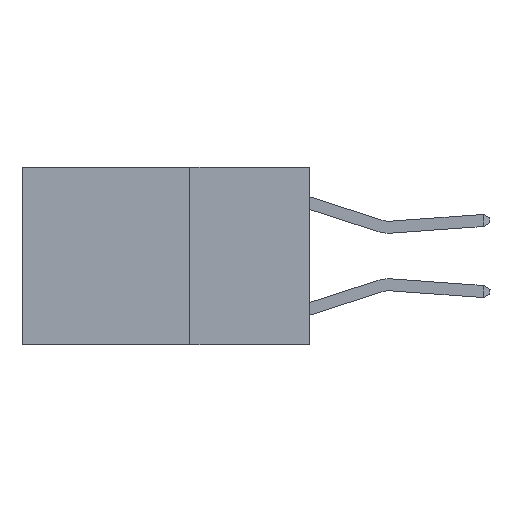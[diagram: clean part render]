
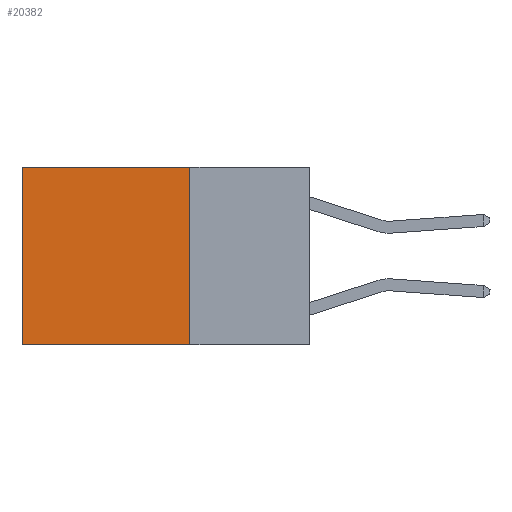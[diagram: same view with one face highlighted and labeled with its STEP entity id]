
A CAD part, left-side view. The second image highlights one B-rep face of the part: STEP entity #20382.
In plain terms, the highlighted planar face has unit normal (-1, 0, 0).
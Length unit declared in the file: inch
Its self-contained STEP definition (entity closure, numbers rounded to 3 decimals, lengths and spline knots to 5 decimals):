
#533 = VERTEX_POINT ( 'NONE', #4999 ) ;
#788 = PLANE ( 'NONE',  #25229 ) ;
#1667 = LINE ( 'NONE', #12451, #21336 ) ;
#1878 = LINE ( 'NONE', #17025, #21306 ) ;
#2861 = LINE ( 'NONE', #4998, #4968 ) ;
#3284 = EDGE_LOOP ( 'NONE', ( #20210, #12112, #8205, #14274 ) ) ;
#3527 = LINE ( 'NONE', #20794, #27763 ) ;
#4647 = EDGE_CURVE ( 'NONE', #10671, #533, #1667, .T. ) ;
#4968 = VECTOR ( 'NONE', #11514, 39.37008 ) ;
#4998 = CARTESIAN_POINT ( 'NONE',  ( 0.2625, 0.6, 0. ) ) ;
#4999 = CARTESIAN_POINT ( 'NONE',  ( 0.2625, 0.25, -0.37 ) ) ;
#8091 = EDGE_CURVE ( 'NONE', #10671, #26003, #1878, .T. ) ;
#8205 = ORIENTED_EDGE ( 'NONE', *, *, #4647, .F. ) ;
#10469 = DIRECTION ( 'NONE',  ( 0., 1., 0. ) ) ;
#10671 = VERTEX_POINT ( 'NONE', #18502 ) ;
#10900 = CARTESIAN_POINT ( 'NONE',  ( 0.2625, 0.6, 0. ) ) ;
#11514 = DIRECTION ( 'NONE',  ( 0., 0., -1. ) ) ;
#12112 = ORIENTED_EDGE ( 'NONE', *, *, #27136, .F. ) ;
#12451 = CARTESIAN_POINT ( 'NONE',  ( 0.2625, 0.25, 0. ) ) ;
#13830 = CARTESIAN_POINT ( 'NONE',  ( 0.2625, 0.25, 0. ) ) ;
#14274 = ORIENTED_EDGE ( 'NONE', *, *, #8091, .T. ) ;
#15683 = FACE_OUTER_BOUND ( 'NONE', #3284, .T. ) ;
#17025 = CARTESIAN_POINT ( 'NONE',  ( 0.2625, 0.25, 0. ) ) ;
#17937 = DIRECTION ( 'NONE',  ( 0., 0., -1. ) ) ;
#18502 = CARTESIAN_POINT ( 'NONE',  ( 0.2625, 0.25, 0. ) ) ;
#20210 = ORIENTED_EDGE ( 'NONE', *, *, #22413, .T. ) ;
#20382 = ADVANCED_FACE ( 'NONE', ( #15683 ), #788, .F. ) ;
#20794 = CARTESIAN_POINT ( 'NONE',  ( 0.2625, 0.25, -0.37 ) ) ;
#21072 = DIRECTION ( 'NONE',  ( 0., 0., -1. ) ) ;
#21224 = CARTESIAN_POINT ( 'NONE',  ( 0.2625, 0.6, -0.37 ) ) ;
#21306 = VECTOR ( 'NONE', #25677, 39.37008 ) ;
#21336 = VECTOR ( 'NONE', #21072, 39.37008 ) ;
#21761 = VERTEX_POINT ( 'NONE', #21224 ) ;
#22413 = EDGE_CURVE ( 'NONE', #26003, #21761, #2861, .T. ) ;
#24586 = DIRECTION ( 'NONE',  ( 1., 0., 0. ) ) ;
#25229 = AXIS2_PLACEMENT_3D ( 'NONE', #13830, #24586, #17937 ) ;
#25677 = DIRECTION ( 'NONE',  ( 0., 1., 0. ) ) ;
#26003 = VERTEX_POINT ( 'NONE', #10900 ) ;
#27136 = EDGE_CURVE ( 'NONE', #533, #21761, #3527, .T. ) ;
#27763 = VECTOR ( 'NONE', #10469, 39.37008 ) ;
